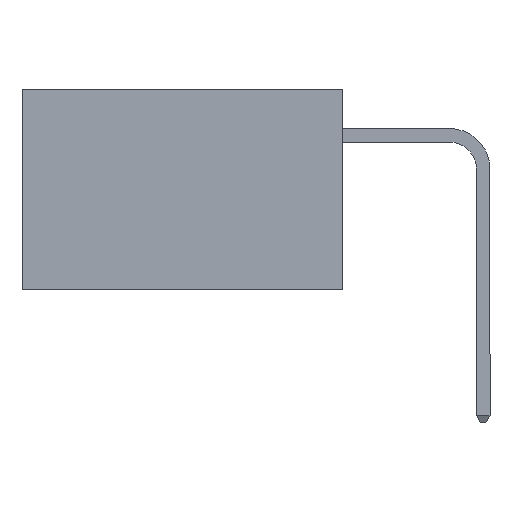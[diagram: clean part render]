
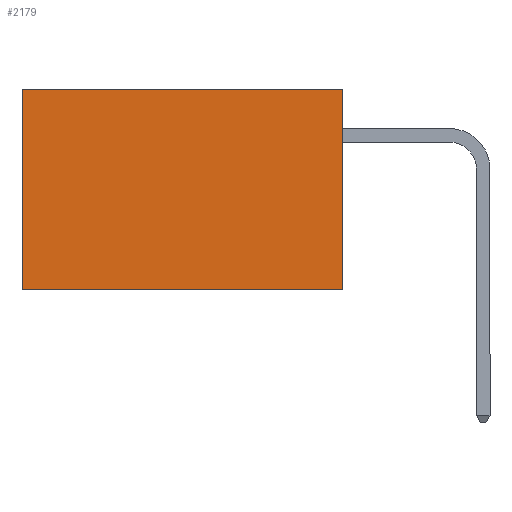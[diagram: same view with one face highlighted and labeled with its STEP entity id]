
A CAD part, left-side view. The second image highlights one B-rep face of the part: STEP entity #2179.
In plain terms, the highlighted planar face has unit normal (-1, 0, 0).
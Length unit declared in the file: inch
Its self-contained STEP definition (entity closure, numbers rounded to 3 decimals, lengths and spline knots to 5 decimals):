
#489 = VERTEX_POINT ( 'NONE', #5768 ) ;
#891 = PLANE ( 'NONE',  #6844 ) ;
#2179 = ADVANCED_FACE ( 'NONE', ( #6957 ), #891, .F. ) ;
#3023 = VERTEX_POINT ( 'NONE', #9709 ) ;
#3288 = CARTESIAN_POINT ( 'NONE',  ( 0.277, 0., 0. ) ) ;
#3306 = VECTOR ( 'NONE', #10299, 39.37008 ) ;
#4060 = ORIENTED_EDGE ( 'NONE', *, *, #7711, .F. ) ;
#4407 = DIRECTION ( 'NONE',  ( 0., 0., -1. ) ) ;
#4423 = LINE ( 'NONE', #3288, #10209 ) ;
#4522 = VECTOR ( 'NONE', #6788, 39.37008 ) ;
#4676 = DIRECTION ( 'NONE',  ( 1., 0., 0. ) ) ;
#4706 = CARTESIAN_POINT ( 'NONE',  ( 0.277, 0., -0.37 ) ) ;
#5748 = VERTEX_POINT ( 'NONE', #6435 ) ;
#5768 = CARTESIAN_POINT ( 'NONE',  ( 0.277, 0.59, 0. ) ) ;
#5833 = EDGE_CURVE ( 'NONE', #3023, #489, #4423, .T. ) ;
#5919 = EDGE_LOOP ( 'NONE', ( #7963, #9903, #4060, #8218 ) ) ;
#6088 = DIRECTION ( 'NONE',  ( 0., 1., 0. ) ) ;
#6435 = CARTESIAN_POINT ( 'NONE',  ( 0.277, 0.59, -0.37 ) ) ;
#6607 = LINE ( 'NONE', #7606, #4522 ) ;
#6788 = DIRECTION ( 'NONE',  ( 0., 0., -1. ) ) ;
#6844 = AXIS2_PLACEMENT_3D ( 'NONE', #4706, #4676, #4407 ) ;
#6957 = FACE_OUTER_BOUND ( 'NONE', #5919, .T. ) ;
#7022 = VECTOR ( 'NONE', #6088, 39.37008 ) ;
#7604 = CARTESIAN_POINT ( 'NONE',  ( 0.277, 0., -0.37 ) ) ;
#7606 = CARTESIAN_POINT ( 'NONE',  ( 0.277, 0., -0.37 ) ) ;
#7711 = EDGE_CURVE ( 'NONE', #3023, #8173, #6607, .T. ) ;
#7963 = ORIENTED_EDGE ( 'NONE', *, *, #8769, .T. ) ;
#8140 = DIRECTION ( 'NONE',  ( 0., 1., 0. ) ) ;
#8173 = VERTEX_POINT ( 'NONE', #9886 ) ;
#8218 = ORIENTED_EDGE ( 'NONE', *, *, #5833, .T. ) ;
#8769 = EDGE_CURVE ( 'NONE', #489, #5748, #9495, .T. ) ;
#9029 = LINE ( 'NONE', #7604, #7022 ) ;
#9495 = LINE ( 'NONE', #9589, #3306 ) ;
#9589 = CARTESIAN_POINT ( 'NONE',  ( 0.277, 0.59, -0.37 ) ) ;
#9709 = CARTESIAN_POINT ( 'NONE',  ( 0.277, 0., 0. ) ) ;
#9886 = CARTESIAN_POINT ( 'NONE',  ( 0.277, 0., -0.37 ) ) ;
#9903 = ORIENTED_EDGE ( 'NONE', *, *, #10155, .F. ) ;
#10155 = EDGE_CURVE ( 'NONE', #8173, #5748, #9029, .T. ) ;
#10209 = VECTOR ( 'NONE', #8140, 39.37008 ) ;
#10299 = DIRECTION ( 'NONE',  ( 0., 0., -1. ) ) ;
